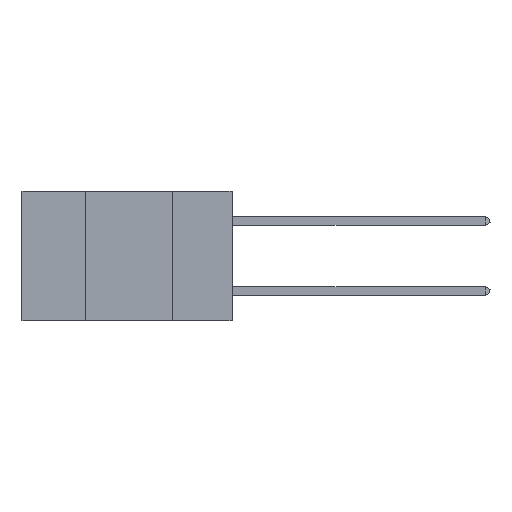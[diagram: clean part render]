
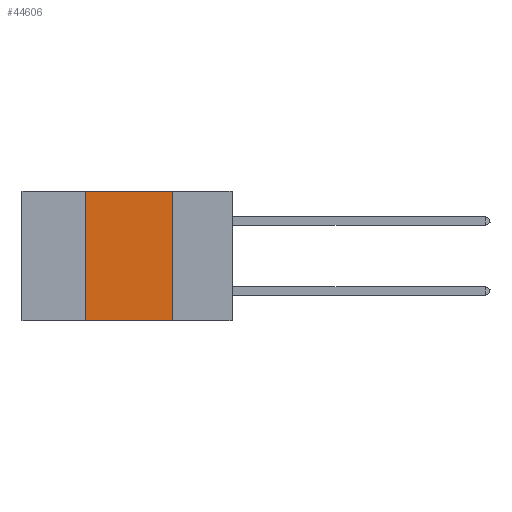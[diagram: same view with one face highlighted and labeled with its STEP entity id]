
A CAD part, left-side view. The second image highlights one B-rep face of the part: STEP entity #44606.
In plain terms, the highlighted planar face has unit normal (-1, 0, 0).
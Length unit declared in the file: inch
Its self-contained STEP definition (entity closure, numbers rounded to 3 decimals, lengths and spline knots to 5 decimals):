
#1112 = EDGE_CURVE ( 'NONE', #46749, #48996, #49835, .T. ) ;
#1242 = DIRECTION ( 'NONE',  ( 0., -1., 0. ) ) ;
#1659 = VERTEX_POINT ( 'NONE', #9212 ) ;
#2154 = CARTESIAN_POINT ( 'NONE',  ( 0., 0.6, -0.37 ) ) ;
#4178 = EDGE_CURVE ( 'NONE', #46749, #1659, #33109, .T. ) ;
#4425 = AXIS2_PLACEMENT_3D ( 'NONE', #34626, #38621, #15333 ) ;
#9212 = CARTESIAN_POINT ( 'NONE',  ( 0., 0.42, 0. ) ) ;
#10107 = DIRECTION ( 'NONE',  ( 0., -1., 0. ) ) ;
#11371 = PLANE ( 'NONE',  #4425 ) ;
#11579 = CARTESIAN_POINT ( 'NONE',  ( 0., 0.17, 0. ) ) ;
#12292 = VECTOR ( 'NONE', #42603, 39.37008 ) ;
#13543 = LINE ( 'NONE', #25733, #22743 ) ;
#15333 = DIRECTION ( 'NONE',  ( 0., 0., -1. ) ) ;
#21884 = EDGE_LOOP ( 'NONE', ( #41985, #44371, #45737, #50202 ) ) ;
#22743 = VECTOR ( 'NONE', #29633, 39.37008 ) ;
#23180 = VECTOR ( 'NONE', #1242, 39.37008 ) ;
#25733 = CARTESIAN_POINT ( 'NONE',  ( 0., 0.17, 0. ) ) ;
#27581 = EDGE_CURVE ( 'NONE', #40893, #48996, #13543, .T. ) ;
#29535 = VECTOR ( 'NONE', #10107, 39.37008 ) ;
#29633 = DIRECTION ( 'NONE',  ( 0., 0., -1. ) ) ;
#30963 = CARTESIAN_POINT ( 'NONE',  ( 0., 0.17, -0.37 ) ) ;
#31252 = CARTESIAN_POINT ( 'NONE',  ( 0., 0.42, 0. ) ) ;
#32352 = LINE ( 'NONE', #48687, #23180 ) ;
#33016 = CARTESIAN_POINT ( 'NONE',  ( 0., 0.42, -0.37 ) ) ;
#33109 = LINE ( 'NONE', #31252, #12292 ) ;
#34626 = CARTESIAN_POINT ( 'NONE',  ( 0., 0.6, 0. ) ) ;
#37760 = EDGE_CURVE ( 'NONE', #1659, #40893, #32352, .T. ) ;
#38621 = DIRECTION ( 'NONE',  ( 1., 0., 0. ) ) ;
#40893 = VERTEX_POINT ( 'NONE', #11579 ) ;
#41985 = ORIENTED_EDGE ( 'NONE', *, *, #27581, .F. ) ;
#42603 = DIRECTION ( 'NONE',  ( 0., 0., 1. ) ) ;
#44371 = ORIENTED_EDGE ( 'NONE', *, *, #37760, .F. ) ;
#44606 = ADVANCED_FACE ( 'NONE', ( #47908 ), #11371, .F. ) ;
#45737 = ORIENTED_EDGE ( 'NONE', *, *, #4178, .F. ) ;
#46749 = VERTEX_POINT ( 'NONE', #33016 ) ;
#47908 = FACE_OUTER_BOUND ( 'NONE', #21884, .T. ) ;
#48687 = CARTESIAN_POINT ( 'NONE',  ( 0., 0.6, 0. ) ) ;
#48996 = VERTEX_POINT ( 'NONE', #30963 ) ;
#49835 = LINE ( 'NONE', #2154, #29535 ) ;
#50202 = ORIENTED_EDGE ( 'NONE', *, *, #1112, .T. ) ;
